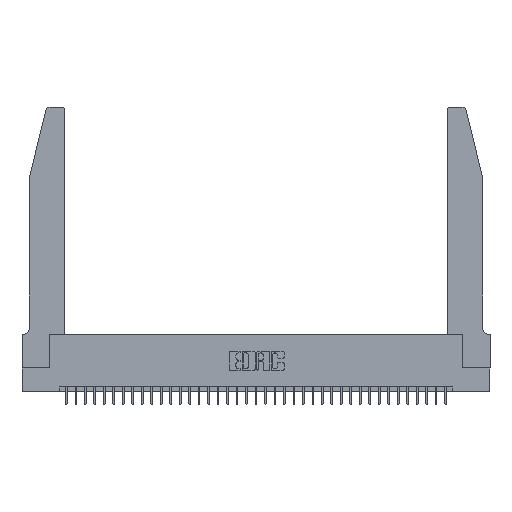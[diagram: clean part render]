
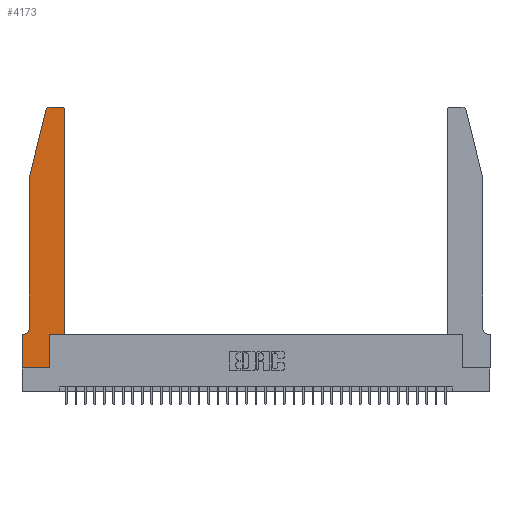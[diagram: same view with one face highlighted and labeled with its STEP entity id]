
A CAD part, top view. The second image highlights one B-rep face of the part: STEP entity #4173.
In plain terms, the highlighted planar face has unit normal (0, 0, 1).
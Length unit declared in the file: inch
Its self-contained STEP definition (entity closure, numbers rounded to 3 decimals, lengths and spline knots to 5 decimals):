
#35 = LINE ( 'NONE', #28608, #16785 ) ;
#241 = LINE ( 'NONE', #32015, #764 ) ;
#764 = VECTOR ( 'NONE', #11717, 39.37008 ) ;
#908 = CARTESIAN_POINT ( 'NONE',  ( 0.4505, 0.35, 0.37 ) ) ;
#942 = DIRECTION ( 'NONE',  ( 0., 0., 1. ) ) ;
#1672 = VERTEX_POINT ( 'NONE', #17507 ) ;
#1699 = FACE_OUTER_BOUND ( 'NONE', #10391, .T. ) ;
#1987 = EDGE_CURVE ( 'NONE', #32455, #1672, #25319, .T. ) ;
#2021 = CARTESIAN_POINT ( 'NONE',  ( 0.0755, 2., 0.37 ) ) ;
#2157 = ORIENTED_EDGE ( 'NONE', *, *, #14783, .T. ) ;
#2313 = VECTOR ( 'NONE', #29733, 39.37008 ) ;
#2314 = DIRECTION ( 'NONE',  ( -1., 0., 0. ) ) ;
#2472 = CARTESIAN_POINT ( 'NONE',  ( 0.25487, 2.72718, 0.37 ) ) ;
#3342 = ORIENTED_EDGE ( 'NONE', *, *, #15205, .T. ) ;
#3428 = DIRECTION ( 'NONE',  ( 1., 0., 0. ) ) ;
#3570 = VECTOR ( 'NONE', #10480, 39.37008 ) ;
#3843 = DIRECTION ( 'NONE',  ( -1., 0., 0. ) ) ;
#4173 = ADVANCED_FACE ( 'NONE', ( #1699 ), #6768, .T. ) ;
#4908 = CARTESIAN_POINT ( 'NONE',  ( 0.0755, 2., 0.37 ) ) ;
#4976 = ORIENTED_EDGE ( 'NONE', *, *, #5952, .T. ) ;
#5009 = CIRCLE ( 'NONE', #7383, 0.03 ) ;
#5321 = CIRCLE ( 'NONE', #16132, 0.03 ) ;
#5755 = LINE ( 'NONE', #14592, #13767 ) ;
#5952 = EDGE_CURVE ( 'NONE', #6348, #14285, #5755, .T. ) ;
#6120 = CARTESIAN_POINT ( 'NONE',  ( 0.0055, 0.42, 0.37 ) ) ;
#6339 = ORIENTED_EDGE ( 'NONE', *, *, #11246, .T. ) ;
#6348 = VERTEX_POINT ( 'NONE', #31980 ) ;
#6768 = PLANE ( 'NONE',  #21498 ) ;
#7383 = AXIS2_PLACEMENT_3D ( 'NONE', #36466, #19536, #16146 ) ;
#7866 = DIRECTION ( 'NONE',  ( 0., -1., 0. ) ) ;
#8636 = VERTEX_POINT ( 'NONE', #29077 ) ;
#10391 = EDGE_LOOP ( 'NONE', ( #31061, #15219, #3342, #29723, #34489, #6339, #28431, #27667, #4976, #36359, #21036, #2157 ) ) ;
#10409 = DIRECTION ( 'NONE',  ( 0., 1., 0. ) ) ;
#10480 = DIRECTION ( 'NONE',  ( 0., -1., 0. ) ) ;
#11153 = LINE ( 'NONE', #24890, #22592 ) ;
#11246 = EDGE_CURVE ( 'NONE', #1672, #8636, #11153, .T. ) ;
#11712 = CARTESIAN_POINT ( 'NONE',  ( 0.0755, 0.42, 0.37 ) ) ;
#11717 = DIRECTION ( 'NONE',  ( -1., 0., 0. ) ) ;
#12595 = VECTOR ( 'NONE', #23407, 39.37008 ) ;
#12810 = VERTEX_POINT ( 'NONE', #17093 ) ;
#13229 = LINE ( 'NONE', #16244, #16842 ) ;
#13767 = VECTOR ( 'NONE', #23247, 39.37008 ) ;
#13910 = VERTEX_POINT ( 'NONE', #31470 ) ;
#14120 = VERTEX_POINT ( 'NONE', #2472 ) ;
#14285 = VERTEX_POINT ( 'NONE', #31153 ) ;
#14592 = CARTESIAN_POINT ( 'NONE',  ( 0.2865, 0.35, 0.37 ) ) ;
#14783 = EDGE_CURVE ( 'NONE', #13910, #12810, #5321, .T. ) ;
#14893 = LINE ( 'NONE', #32563, #2313 ) ;
#14910 = VERTEX_POINT ( 'NONE', #21120 ) ;
#15205 = EDGE_CURVE ( 'NONE', #14120, #29681, #35, .T. ) ;
#15219 = ORIENTED_EDGE ( 'NONE', *, *, #23751, .T. ) ;
#15399 = VERTEX_POINT ( 'NONE', #24447 ) ;
#15989 = EDGE_CURVE ( 'NONE', #29681, #32455, #33439, .T. ) ;
#16132 = AXIS2_PLACEMENT_3D ( 'NONE', #32206, #34315, #3428 ) ;
#16146 = DIRECTION ( 'NONE',  ( 1., 0., 0. ) ) ;
#16244 = CARTESIAN_POINT ( 'NONE',  ( 0.4505, 0.35, 0.37 ) ) ;
#16785 = VECTOR ( 'NONE', #37095, 39.37008 ) ;
#16842 = VECTOR ( 'NONE', #10409, 39.37008 ) ;
#17093 = CARTESIAN_POINT ( 'NONE',  ( 0.4205, 2.75, 0.37 ) ) ;
#17507 = CARTESIAN_POINT ( 'NONE',  ( 0.0055, 0.35, 0.37 ) ) ;
#17687 = EDGE_CURVE ( 'NONE', #15399, #6348, #35063, .T. ) ;
#19536 = DIRECTION ( 'NONE',  ( 0., 0., 1. ) ) ;
#21036 = ORIENTED_EDGE ( 'NONE', *, *, #32373, .T. ) ;
#21120 = CARTESIAN_POINT ( 'NONE',  ( 0.284, 2.75, 0.37 ) ) ;
#21498 = AXIS2_PLACEMENT_3D ( 'NONE', #35365, #942, #27467 ) ;
#22592 = VECTOR ( 'NONE', #2314, 39.37008 ) ;
#23247 = DIRECTION ( 'NONE',  ( 0., 1., 0. ) ) ;
#23407 = DIRECTION ( 'NONE',  ( 1., 0., 0. ) ) ;
#23751 = EDGE_CURVE ( 'NONE', #14910, #14120, #5009, .T. ) ;
#23832 = EDGE_CURVE ( 'NONE', #8636, #15399, #27991, .T. ) ;
#24220 = VECTOR ( 'NONE', #7866, 39.37008 ) ;
#24447 = CARTESIAN_POINT ( 'NONE',  ( 0., 0., 0.37 ) ) ;
#24890 = CARTESIAN_POINT ( 'NONE',  ( 0.0755, 0.35, 0.37 ) ) ;
#25319 = CIRCLE ( 'NONE', #27100, 0.07 ) ;
#27100 = AXIS2_PLACEMENT_3D ( 'NONE', #6120, #31702, #3843 ) ;
#27467 = DIRECTION ( 'NONE',  ( 1., 0., 0. ) ) ;
#27667 = ORIENTED_EDGE ( 'NONE', *, *, #17687, .T. ) ;
#27991 = LINE ( 'NONE', #31179, #24220 ) ;
#28431 = ORIENTED_EDGE ( 'NONE', *, *, #23832, .T. ) ;
#28608 = CARTESIAN_POINT ( 'NONE',  ( 0.0755, 2., 0.37 ) ) ;
#28782 = EDGE_CURVE ( 'NONE', #14285, #31307, #14893, .T. ) ;
#29077 = CARTESIAN_POINT ( 'NONE',  ( 0., 0.35, 0.37 ) ) ;
#29681 = VERTEX_POINT ( 'NONE', #4908 ) ;
#29723 = ORIENTED_EDGE ( 'NONE', *, *, #15989, .T. ) ;
#29733 = DIRECTION ( 'NONE',  ( 1., 0., 0. ) ) ;
#31061 = ORIENTED_EDGE ( 'NONE', *, *, #35907, .T. ) ;
#31153 = CARTESIAN_POINT ( 'NONE',  ( 0.2865, 0.35, 0.37 ) ) ;
#31179 = CARTESIAN_POINT ( 'NONE',  ( 0., 0., 0.37 ) ) ;
#31307 = VERTEX_POINT ( 'NONE', #908 ) ;
#31470 = CARTESIAN_POINT ( 'NONE',  ( 0.4505, 2.72, 0.37 ) ) ;
#31702 = DIRECTION ( 'NONE',  ( 0., 0., -1. ) ) ;
#31980 = CARTESIAN_POINT ( 'NONE',  ( 0.2865, 0., 0.37 ) ) ;
#32015 = CARTESIAN_POINT ( 'NONE',  ( 0.2605, 2.75, 0.37 ) ) ;
#32206 = CARTESIAN_POINT ( 'NONE',  ( 0.4205, 2.72, 0.37 ) ) ;
#32373 = EDGE_CURVE ( 'NONE', #31307, #13910, #13229, .T. ) ;
#32455 = VERTEX_POINT ( 'NONE', #11712 ) ;
#32563 = CARTESIAN_POINT ( 'NONE',  ( 0.4505, 0.35, 0.37 ) ) ;
#32609 = CARTESIAN_POINT ( 'NONE',  ( 0., 0., 0.37 ) ) ;
#33439 = LINE ( 'NONE', #2021, #3570 ) ;
#34315 = DIRECTION ( 'NONE',  ( 0., 0., 1. ) ) ;
#34489 = ORIENTED_EDGE ( 'NONE', *, *, #1987, .T. ) ;
#35063 = LINE ( 'NONE', #32609, #12595 ) ;
#35365 = CARTESIAN_POINT ( 'NONE',  ( 0., 0.35, 0.37 ) ) ;
#35907 = EDGE_CURVE ( 'NONE', #12810, #14910, #241, .T. ) ;
#36359 = ORIENTED_EDGE ( 'NONE', *, *, #28782, .T. ) ;
#36466 = CARTESIAN_POINT ( 'NONE',  ( 0.284, 2.72, 0.37 ) ) ;
#37095 = DIRECTION ( 'NONE',  ( -0.239, -0.971, 0. ) ) ;
